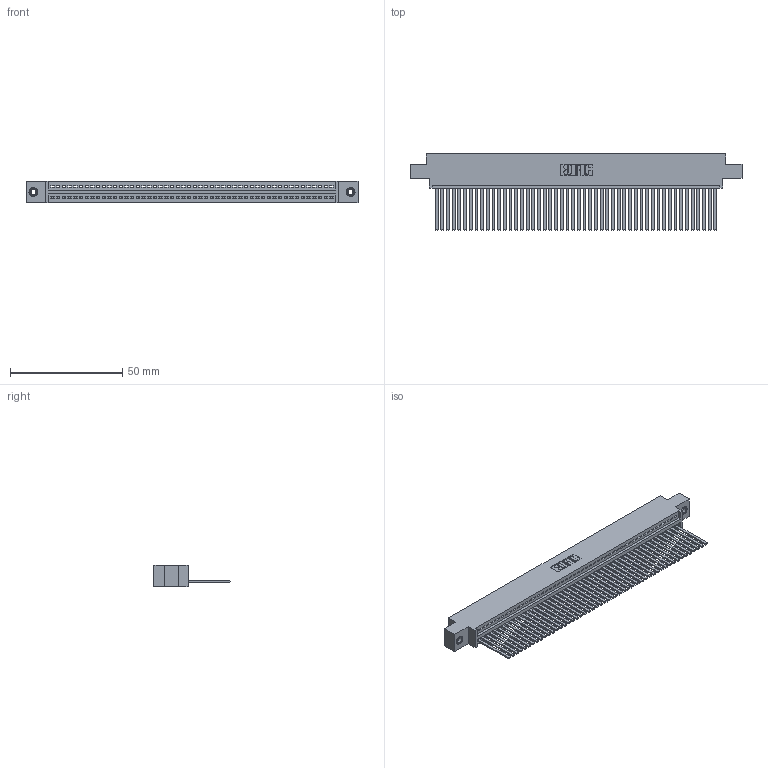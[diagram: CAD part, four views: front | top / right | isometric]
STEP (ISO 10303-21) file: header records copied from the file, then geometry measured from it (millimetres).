
FILE_DESCRIPTION (( 'STEP AP203' ), '1' );
FILE_NAME ('395-050-544-608.STEP', '2018-11-20T09:35:08', ( '' ), ( '' ), 'SwSTEP 2.0', 'SolidWorks 2016', '' );
FILE_SCHEMA (( 'CONFIG_CONTROL_DESIGN' ));
Length unit declared in the file: inch
Products named in the file (4): 395-050-544-608; 345 Part_0.170 Offset - 0.156 Dia-TI; 345-250-001_345-250-003-102; 345-292-001_345-293-144
Assembly tree (53 placements, depth 2):
  395-050-544-608
    345 Part_0.170 Offset - 0.156 Dia-TI
    345-292-001_345-293-144  x50
    345-250-001_345-250-003-102  x2
Bounding box: 148.21 x 33.96 x 9.4 mm (x, y, z)
Volume: 14601.7 mm3; surface area: 21397.2 mm2
Topology: 53 solids, 53 shells, 2790 faces, 8389 edges, 5518 vertices
Faces by surface type: plane 1916, cylinder 858, cone 12, torus 4
Entity records: 37688 total; most frequent: CARTESIAN_POINT 6509, ORIENTED_EDGE 6486, DIRECTION 5697, EDGE_CURVE 3243, VECTOR 2895, LINE 2895, VERTEX_POINT 2156, AXIS2_PLACEMENT_3D 1401
